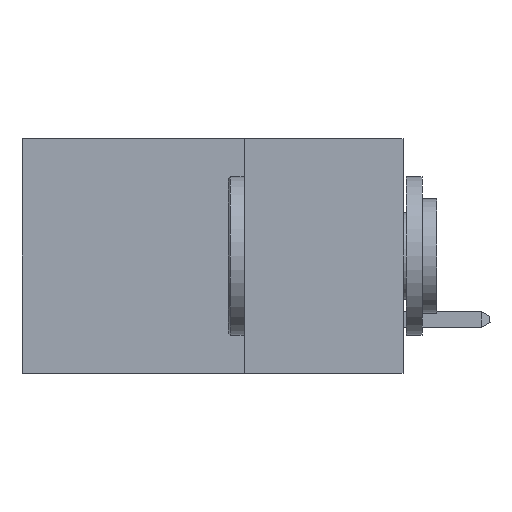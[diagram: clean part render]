
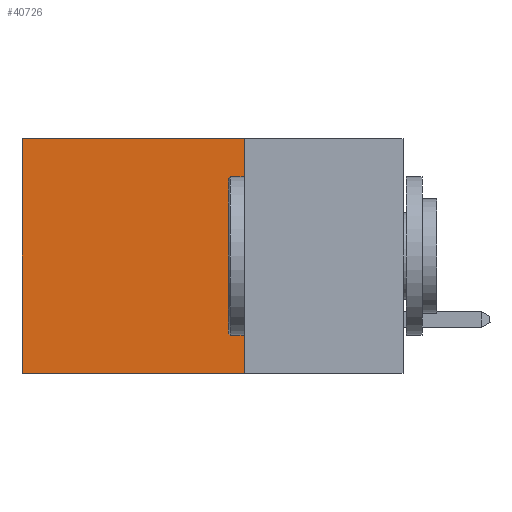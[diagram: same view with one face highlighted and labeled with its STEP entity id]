
A CAD part, left-side view. The second image highlights one B-rep face of the part: STEP entity #40726.
In plain terms, the highlighted planar face has unit normal (-1, 0, 0).
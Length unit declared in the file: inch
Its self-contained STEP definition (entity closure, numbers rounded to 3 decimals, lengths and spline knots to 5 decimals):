
#2948 = ORIENTED_EDGE ( 'NONE', *, *, #17061, .F. ) ;
#5087 = LINE ( 'NONE', #7967, #10755 ) ;
#6477 = VERTEX_POINT ( 'NONE', #39052 ) ;
#6568 = FACE_OUTER_BOUND ( 'NONE', #30435, .T. ) ;
#6717 = CARTESIAN_POINT ( 'NONE',  ( 0.2875, 0.6, 0. ) ) ;
#6722 = ORIENTED_EDGE ( 'NONE', *, *, #32100, .T. ) ;
#7967 = CARTESIAN_POINT ( 'NONE',  ( 0.2875, 0.25, 0. ) ) ;
#8272 = VECTOR ( 'NONE', #10931, 39.37008 ) ;
#9186 = VECTOR ( 'NONE', #21440, 39.37008 ) ;
#10701 = VERTEX_POINT ( 'NONE', #25414 ) ;
#10755 = VECTOR ( 'NONE', #43910, 39.37008 ) ;
#10931 = DIRECTION ( 'NONE',  ( 0., 1., 0. ) ) ;
#14233 = DIRECTION ( 'NONE',  ( 0., 1., 0. ) ) ;
#15886 = EDGE_CURVE ( 'NONE', #21476, #10701, #34176, .T. ) ;
#16887 = ORIENTED_EDGE ( 'NONE', *, *, #15886, .T. ) ;
#17061 = EDGE_CURVE ( 'NONE', #6477, #17555, #5087, .T. ) ;
#17357 = DIRECTION ( 'NONE',  ( 1., 0., 0. ) ) ;
#17555 = VERTEX_POINT ( 'NONE', #32376 ) ;
#20903 = CARTESIAN_POINT ( 'NONE',  ( 0.2875, 0.25, 0. ) ) ;
#21440 = DIRECTION ( 'NONE',  ( 0., 0., -1. ) ) ;
#21476 = VERTEX_POINT ( 'NONE', #36325 ) ;
#23681 = VECTOR ( 'NONE', #14233, 39.37008 ) ;
#24684 = DIRECTION ( 'NONE',  ( 0., 0., -1. ) ) ;
#25414 = CARTESIAN_POINT ( 'NONE',  ( 0.2875, 0.6, -0.37 ) ) ;
#25730 = CARTESIAN_POINT ( 'NONE',  ( 0.2875, 0.25, -0.37 ) ) ;
#29798 = ORIENTED_EDGE ( 'NONE', *, *, #45390, .F. ) ;
#30018 = AXIS2_PLACEMENT_3D ( 'NONE', #46492, #17357, #24684 ) ;
#30435 = EDGE_LOOP ( 'NONE', ( #16887, #29798, #2948, #6722 ) ) ;
#31564 = LINE ( 'NONE', #25730, #8272 ) ;
#32100 = EDGE_CURVE ( 'NONE', #6477, #21476, #43599, .T. ) ;
#32376 = CARTESIAN_POINT ( 'NONE',  ( 0.2875, 0.25, -0.37 ) ) ;
#34176 = LINE ( 'NONE', #6717, #9186 ) ;
#35836 = PLANE ( 'NONE',  #30018 ) ;
#36325 = CARTESIAN_POINT ( 'NONE',  ( 0.2875, 0.6, 0. ) ) ;
#39052 = CARTESIAN_POINT ( 'NONE',  ( 0.2875, 0.25, 0. ) ) ;
#40726 = ADVANCED_FACE ( 'NONE', ( #6568 ), #35836, .F. ) ;
#43599 = LINE ( 'NONE', #20903, #23681 ) ;
#43910 = DIRECTION ( 'NONE',  ( 0., 0., -1. ) ) ;
#45390 = EDGE_CURVE ( 'NONE', #17555, #10701, #31564, .T. ) ;
#46492 = CARTESIAN_POINT ( 'NONE',  ( 0.2875, 0.25, 0. ) ) ;
